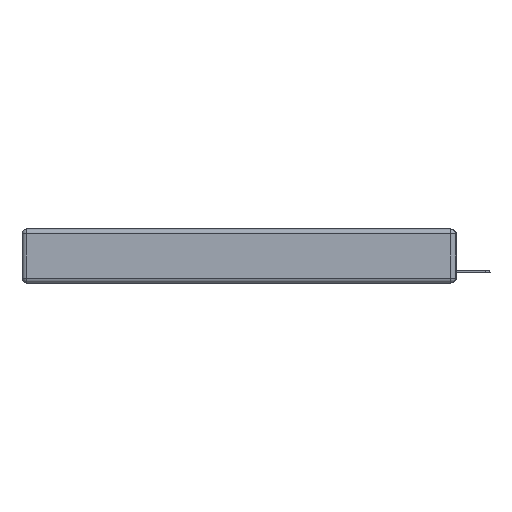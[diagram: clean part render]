
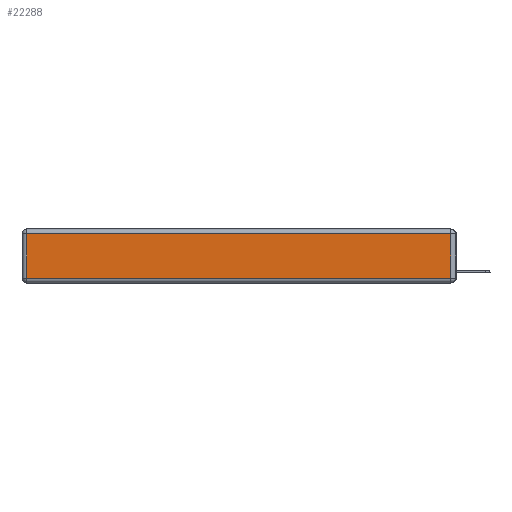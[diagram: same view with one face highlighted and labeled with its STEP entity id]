
A CAD part, left-side view. The second image highlights one B-rep face of the part: STEP entity #22288.
In plain terms, the highlighted planar face has unit normal (-1, 0, 0).
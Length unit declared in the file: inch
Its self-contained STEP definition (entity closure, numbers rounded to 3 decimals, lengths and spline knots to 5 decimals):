
#294 = VECTOR ( 'NONE', #3669, 39.37008 ) ;
#705 = CARTESIAN_POINT ( 'NONE',  ( 0., 2.72, -0.03 ) ) ;
#947 = FACE_OUTER_BOUND ( 'NONE', #24432, .T. ) ;
#1271 = VECTOR ( 'NONE', #7078, 39.37008 ) ;
#1619 = VERTEX_POINT ( 'NONE', #7297 ) ;
#1697 = DIRECTION ( 'NONE',  ( 0., 0., 1. ) ) ;
#3669 = DIRECTION ( 'NONE',  ( 0., 0., -1. ) ) ;
#6456 = VECTOR ( 'NONE', #11929, 39.37008 ) ;
#7078 = DIRECTION ( 'NONE',  ( 0., -1., 0. ) ) ;
#7252 = AXIS2_PLACEMENT_3D ( 'NONE', #22847, #13030, #1697 ) ;
#7297 = CARTESIAN_POINT ( 'NONE',  ( 0., 0.03, -0.03 ) ) ;
#7579 = LINE ( 'NONE', #15488, #294 ) ;
#8838 = VERTEX_POINT ( 'NONE', #21537 ) ;
#10051 = LINE ( 'NONE', #19481, #6456 ) ;
#10599 = CARTESIAN_POINT ( 'NONE',  ( 0., 2.75, -0.03 ) ) ;
#10977 = LINE ( 'NONE', #16632, #1271 ) ;
#11929 = DIRECTION ( 'NONE',  ( 0., 0., 1. ) ) ;
#12744 = VERTEX_POINT ( 'NONE', #16367 ) ;
#13030 = DIRECTION ( 'NONE',  ( -1., 0., 0. ) ) ;
#15488 = CARTESIAN_POINT ( 'NONE',  ( 0., 2.72, -0.343 ) ) ;
#16367 = CARTESIAN_POINT ( 'NONE',  ( 0., 2.72, -0.313 ) ) ;
#16632 = CARTESIAN_POINT ( 'NONE',  ( 0., 0., -0.313 ) ) ;
#17185 = ORIENTED_EDGE ( 'NONE', *, *, #19732, .T. ) ;
#18066 = EDGE_CURVE ( 'NONE', #12744, #8838, #10977, .T. ) ;
#18333 = PLANE ( 'NONE',  #7252 ) ;
#19205 = VECTOR ( 'NONE', #23929, 39.37008 ) ;
#19481 = CARTESIAN_POINT ( 'NONE',  ( 0., 0.03, -0.343 ) ) ;
#19536 = ORIENTED_EDGE ( 'NONE', *, *, #18066, .T. ) ;
#19732 = EDGE_CURVE ( 'NONE', #1619, #24700, #24304, .T. ) ;
#19854 = ORIENTED_EDGE ( 'NONE', *, *, #24429, .T. ) ;
#19888 = EDGE_CURVE ( 'NONE', #24700, #12744, #7579, .T. ) ;
#21537 = CARTESIAN_POINT ( 'NONE',  ( 0., 0.03, -0.313 ) ) ;
#22288 = ADVANCED_FACE ( 'NONE', ( #947 ), #18333, .T. ) ;
#22847 = CARTESIAN_POINT ( 'NONE',  ( 0., 0., -0.343 ) ) ;
#23266 = ORIENTED_EDGE ( 'NONE', *, *, #19888, .T. ) ;
#23929 = DIRECTION ( 'NONE',  ( 0., 1., 0. ) ) ;
#24304 = LINE ( 'NONE', #10599, #19205 ) ;
#24429 = EDGE_CURVE ( 'NONE', #8838, #1619, #10051, .T. ) ;
#24432 = EDGE_LOOP ( 'NONE', ( #19536, #19854, #17185, #23266 ) ) ;
#24700 = VERTEX_POINT ( 'NONE', #705 ) ;
